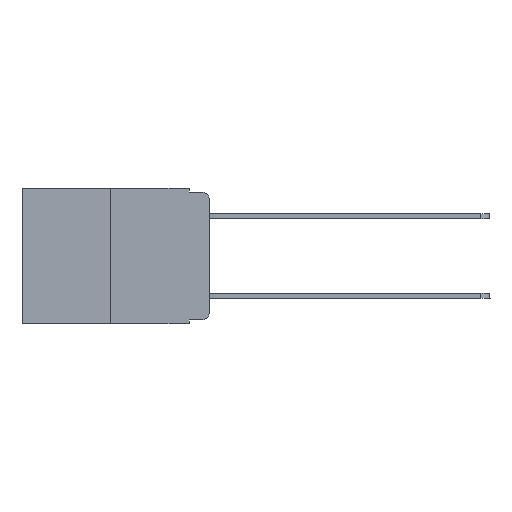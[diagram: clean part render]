
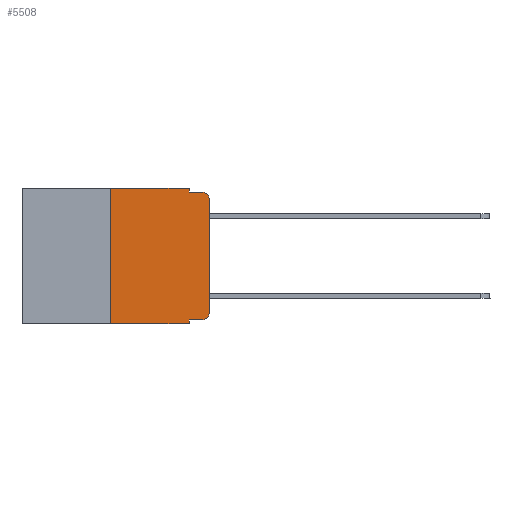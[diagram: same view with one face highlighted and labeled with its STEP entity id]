
A CAD part, left-side view. The second image highlights one B-rep face of the part: STEP entity #5508.
In plain terms, the highlighted planar face has unit normal (-1, 0, 0).
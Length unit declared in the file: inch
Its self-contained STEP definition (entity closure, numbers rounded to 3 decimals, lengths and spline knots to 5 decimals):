
#61 = DIRECTION ( 'NONE',  ( 0., 0., -1. ) ) ;
#287 = DIRECTION ( 'NONE',  ( 0., 0., -1. ) ) ;
#299 = CARTESIAN_POINT ( 'NONE',  ( 0., 0.02, -0.313 ) ) ;
#385 = CARTESIAN_POINT ( 'NONE',  ( 0., 0.25, 0. ) ) ;
#832 = CARTESIAN_POINT ( 'NONE',  ( 0., 0.02, -0.333 ) ) ;
#1412 = DIRECTION ( 'NONE',  ( 0., -1., 0. ) ) ;
#1693 = DIRECTION ( 'NONE',  ( 0., 0., -1. ) ) ;
#1710 = CARTESIAN_POINT ( 'NONE',  ( 0., 0.02, -0.03 ) ) ;
#1874 = EDGE_CURVE ( 'NONE', #19499, #10848, #6607, .T. ) ;
#2553 = EDGE_CURVE ( 'NONE', #10848, #14389, #16930, .T. ) ;
#3054 = VERTEX_POINT ( 'NONE', #20655 ) ;
#3137 = ORIENTED_EDGE ( 'NONE', *, *, #16890, .T. ) ;
#3346 = ORIENTED_EDGE ( 'NONE', *, *, #9028, .T. ) ;
#3357 = CARTESIAN_POINT ( 'NONE',  ( 0., 0.051, -0.343 ) ) ;
#3544 = ORIENTED_EDGE ( 'NONE', *, *, #16461, .T. ) ;
#3559 = CIRCLE ( 'NONE', #8823, 0.02 ) ;
#3893 = EDGE_CURVE ( 'NONE', #3054, #5603, #20058, .T. ) ;
#4418 = DIRECTION ( 'NONE',  ( 0., -1., 0. ) ) ;
#5027 = CARTESIAN_POINT ( 'NONE',  ( 0., 0.051, 0. ) ) ;
#5248 = DIRECTION ( 'NONE',  ( -1., 0., 0. ) ) ;
#5508 = ADVANCED_FACE ( 'NONE', ( #15092 ), #6875, .F. ) ;
#5603 = VERTEX_POINT ( 'NONE', #3357 ) ;
#5898 = VERTEX_POINT ( 'NONE', #15171 ) ;
#5995 = DIRECTION ( 'NONE',  ( 0., 0., 1. ) ) ;
#6264 = CARTESIAN_POINT ( 'NONE',  ( 0., 0.051, -0.333 ) ) ;
#6333 = CARTESIAN_POINT ( 'NONE',  ( 0., 0.25, -0.343 ) ) ;
#6607 = LINE ( 'NONE', #13290, #7094 ) ;
#6875 = PLANE ( 'NONE',  #11449 ) ;
#6967 = CARTESIAN_POINT ( 'NONE',  ( 0., 0.051, 0. ) ) ;
#7094 = VECTOR ( 'NONE', #19990, 39.37008 ) ;
#7250 = VECTOR ( 'NONE', #5995, 39.37008 ) ;
#7268 = CIRCLE ( 'NONE', #18438, 0.02 ) ;
#8087 = ORIENTED_EDGE ( 'NONE', *, *, #1874, .F. ) ;
#8165 = ORIENTED_EDGE ( 'NONE', *, *, #20431, .F. ) ;
#8187 = DIRECTION ( 'NONE',  ( 0., -1., 0. ) ) ;
#8415 = DIRECTION ( 'NONE',  ( -1., 0., 0. ) ) ;
#8438 = DIRECTION ( 'NONE',  ( 0., 0., -1. ) ) ;
#8823 = AXIS2_PLACEMENT_3D ( 'NONE', #1710, #8415, #61 ) ;
#8842 = ORIENTED_EDGE ( 'NONE', *, *, #3893, .F. ) ;
#9028 = EDGE_CURVE ( 'NONE', #5898, #16385, #3559, .T. ) ;
#9942 = DIRECTION ( 'NONE',  ( 1., 0., 0. ) ) ;
#10030 = LINE ( 'NONE', #16718, #11092 ) ;
#10370 = VERTEX_POINT ( 'NONE', #14016 ) ;
#10376 = VECTOR ( 'NONE', #4418, 39.37008 ) ;
#10517 = VECTOR ( 'NONE', #8438, 39.37008 ) ;
#10848 = VERTEX_POINT ( 'NONE', #385 ) ;
#10913 = ORIENTED_EDGE ( 'NONE', *, *, #15599, .F. ) ;
#11075 = VECTOR ( 'NONE', #15499, 39.37008 ) ;
#11092 = VECTOR ( 'NONE', #1693, 39.37008 ) ;
#11148 = CARTESIAN_POINT ( 'NONE',  ( 0., 0., 0. ) ) ;
#11406 = LINE ( 'NONE', #6264, #19529 ) ;
#11449 = AXIS2_PLACEMENT_3D ( 'NONE', #18169, #9942, #287 ) ;
#12504 = CARTESIAN_POINT ( 'NONE',  ( 0., 0.02, -0.01 ) ) ;
#13290 = CARTESIAN_POINT ( 'NONE',  ( 0., 0.25, 0. ) ) ;
#13449 = DIRECTION ( 'NONE',  ( 0., 0., -1. ) ) ;
#13528 = CARTESIAN_POINT ( 'NONE',  ( 0., 0.473, -0.343 ) ) ;
#14016 = CARTESIAN_POINT ( 'NONE',  ( 0., 0.051, -0.01 ) ) ;
#14389 = VERTEX_POINT ( 'NONE', #6967 ) ;
#14647 = VERTEX_POINT ( 'NONE', #16361 ) ;
#14943 = ORIENTED_EDGE ( 'NONE', *, *, #2553, .F. ) ;
#14968 = LINE ( 'NONE', #13528, #15338 ) ;
#15092 = FACE_OUTER_BOUND ( 'NONE', #17596, .T. ) ;
#15166 = ORIENTED_EDGE ( 'NONE', *, *, #21054, .T. ) ;
#15171 = CARTESIAN_POINT ( 'NONE',  ( 0., 0., -0.03 ) ) ;
#15280 = CARTESIAN_POINT ( 'NONE',  ( 0., 0.473, 0. ) ) ;
#15338 = VECTOR ( 'NONE', #8187, 39.37008 ) ;
#15499 = DIRECTION ( 'NONE',  ( 0., -1., 0. ) ) ;
#15583 = ORIENTED_EDGE ( 'NONE', *, *, #20911, .T. ) ;
#15599 = EDGE_CURVE ( 'NONE', #14389, #10370, #10030, .T. ) ;
#16361 = CARTESIAN_POINT ( 'NONE',  ( 0., 0., -0.313 ) ) ;
#16385 = VERTEX_POINT ( 'NONE', #12504 ) ;
#16461 = EDGE_CURVE ( 'NONE', #3054, #18579, #11406, .T. ) ;
#16718 = CARTESIAN_POINT ( 'NONE',  ( 0., 0.051, 0. ) ) ;
#16890 = EDGE_CURVE ( 'NONE', #19499, #5603, #14968, .T. ) ;
#16930 = LINE ( 'NONE', #15280, #11075 ) ;
#17596 = EDGE_LOOP ( 'NONE', ( #15166, #3346, #8165, #10913, #14943, #8087, #3137, #8842, #3544, #15583 ) ) ;
#17631 = LINE ( 'NONE', #11148, #7250 ) ;
#17813 = LINE ( 'NONE', #18015, #10376 ) ;
#18015 = CARTESIAN_POINT ( 'NONE',  ( 0., 0.051, -0.01 ) ) ;
#18169 = CARTESIAN_POINT ( 'NONE',  ( 0., 0.473, 0. ) ) ;
#18438 = AXIS2_PLACEMENT_3D ( 'NONE', #299, #5248, #13449 ) ;
#18579 = VERTEX_POINT ( 'NONE', #832 ) ;
#19499 = VERTEX_POINT ( 'NONE', #6333 ) ;
#19529 = VECTOR ( 'NONE', #1412, 39.37008 ) ;
#19990 = DIRECTION ( 'NONE',  ( 0., 0., 1. ) ) ;
#20058 = LINE ( 'NONE', #5027, #10517 ) ;
#20431 = EDGE_CURVE ( 'NONE', #10370, #16385, #17813, .T. ) ;
#20655 = CARTESIAN_POINT ( 'NONE',  ( 0., 0.051, -0.333 ) ) ;
#20911 = EDGE_CURVE ( 'NONE', #18579, #14647, #7268, .T. ) ;
#21054 = EDGE_CURVE ( 'NONE', #14647, #5898, #17631, .T. ) ;
